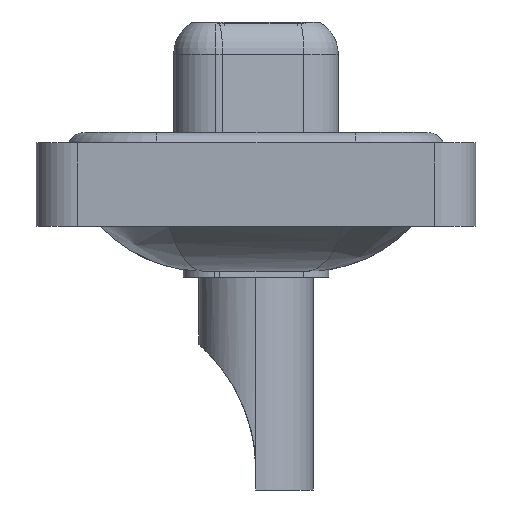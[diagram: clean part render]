
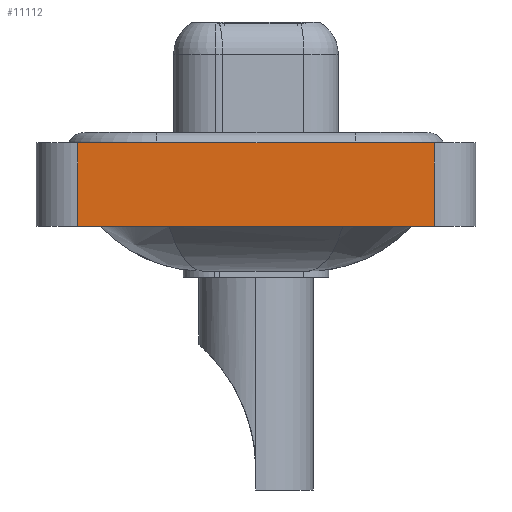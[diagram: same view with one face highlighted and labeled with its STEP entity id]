
A CAD part, left-side view. The second image highlights one B-rep face of the part: STEP entity #11112.
In plain terms, the highlighted planar face has unit normal (-1, 0, 0).
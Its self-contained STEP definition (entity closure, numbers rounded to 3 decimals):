
#797 = PLANE ( 'NONE',  #15142 ) ;
#954 = LINE ( 'NONE', #2701, #9320 ) ;
#1121 = CARTESIAN_POINT ( 'NONE',  ( -7.3, -8.55, -3.6 ) ) ;
#1521 = LINE ( 'NONE', #12769, #15595 ) ;
#1989 = CARTESIAN_POINT ( 'NONE',  ( -7.3, -8.55, -3.6 ) ) ;
#2022 = EDGE_CURVE ( 'NONE', #12972, #6551, #1521, .T. ) ;
#2266 = ORIENTED_EDGE ( 'NONE', *, *, #6057, .F. ) ;
#2701 = CARTESIAN_POINT ( 'NONE',  ( -7.3, 8.55, -3.6 ) ) ;
#3262 = ORIENTED_EDGE ( 'NONE', *, *, #2022, .T. ) ;
#3429 = LINE ( 'NONE', #9336, #15005 ) ;
#3725 = CARTESIAN_POINT ( 'NONE',  ( -7.3, 8.55, 0.4 ) ) ;
#4398 = ORIENTED_EDGE ( 'NONE', *, *, #14475, .F. ) ;
#5865 = DIRECTION ( 'NONE',  ( 0., 0., 1. ) ) ;
#5948 = EDGE_CURVE ( 'NONE', #8547, #12972, #3429, .T. ) ;
#5957 = DIRECTION ( 'NONE',  ( 0., 0., 1. ) ) ;
#6000 = CARTESIAN_POINT ( 'NONE',  ( -7.3, -8.55, 0.4 ) ) ;
#6057 = EDGE_CURVE ( 'NONE', #15163, #6551, #12161, .T. ) ;
#6173 = CARTESIAN_POINT ( 'NONE',  ( -7.3, 8.55, -3.6 ) ) ;
#6551 = VERTEX_POINT ( 'NONE', #12711 ) ;
#6712 = ORIENTED_EDGE ( 'NONE', *, *, #5948, .T. ) ;
#7106 = FACE_OUTER_BOUND ( 'NONE', #8031, .T. ) ;
#8031 = EDGE_LOOP ( 'NONE', ( #3262, #2266, #4398, #6712 ) ) ;
#8547 = VERTEX_POINT ( 'NONE', #6173 ) ;
#8677 = DIRECTION ( 'NONE',  ( 0., -1., 0. ) ) ;
#9320 = VECTOR ( 'NONE', #5865, 1000. ) ;
#9336 = CARTESIAN_POINT ( 'NONE',  ( -7.3, -8.55, -3.6 ) ) ;
#11112 = ADVANCED_FACE ( 'NONE', ( #7106 ), #797, .T. ) ;
#11882 = DIRECTION ( 'NONE',  ( -1., 0., 0. ) ) ;
#12161 = LINE ( 'NONE', #6000, #14714 ) ;
#12711 = CARTESIAN_POINT ( 'NONE',  ( -7.3, -8.55, 0.4 ) ) ;
#12769 = CARTESIAN_POINT ( 'NONE',  ( -7.3, -8.55, -3.6 ) ) ;
#12972 = VERTEX_POINT ( 'NONE', #1989 ) ;
#14303 = DIRECTION ( 'NONE',  ( 0., -1., 0. ) ) ;
#14475 = EDGE_CURVE ( 'NONE', #8547, #15163, #954, .T. ) ;
#14714 = VECTOR ( 'NONE', #8677, 1000. ) ;
#15005 = VECTOR ( 'NONE', #14303, 1000. ) ;
#15142 = AXIS2_PLACEMENT_3D ( 'NONE', #1121, #11882, #5957 ) ;
#15163 = VERTEX_POINT ( 'NONE', #3725 ) ;
#15306 = DIRECTION ( 'NONE',  ( 0., 0., 1. ) ) ;
#15595 = VECTOR ( 'NONE', #15306, 1000. ) ;
